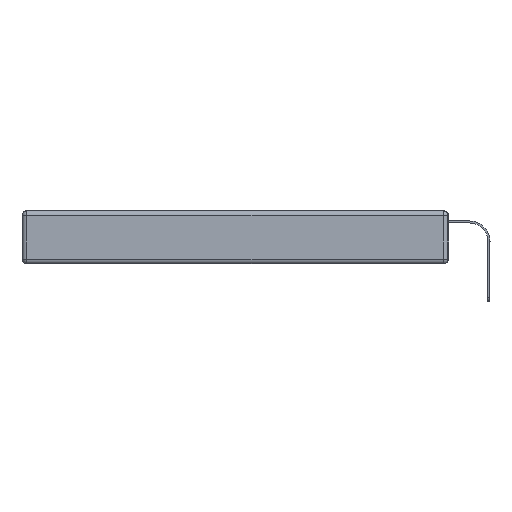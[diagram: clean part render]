
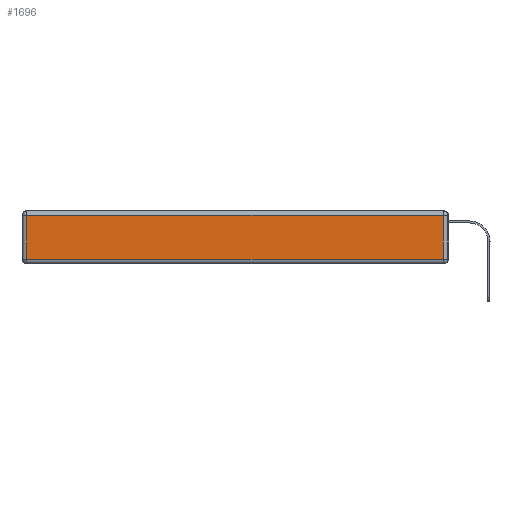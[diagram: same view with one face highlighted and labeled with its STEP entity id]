
A CAD part, left-side view. The second image highlights one B-rep face of the part: STEP entity #1696.
In plain terms, the highlighted planar face has unit normal (-1, 0, 0).
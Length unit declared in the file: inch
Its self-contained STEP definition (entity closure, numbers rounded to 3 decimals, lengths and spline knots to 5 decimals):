
#99 = VECTOR ( 'NONE', #16522, 39.37008 ) ;
#902 = VERTEX_POINT ( 'NONE', #2886 ) ;
#1073 = VECTOR ( 'NONE', #4844, 39.37008 ) ;
#1696 = ADVANCED_FACE ( 'NONE', ( #3199 ), #6491, .T. ) ;
#2133 = ORIENTED_EDGE ( 'NONE', *, *, #19074, .T. ) ;
#2134 = ORIENTED_EDGE ( 'NONE', *, *, #17268, .T. ) ;
#2862 = LINE ( 'NONE', #7171, #3297 ) ;
#2886 = CARTESIAN_POINT ( 'NONE',  ( 0., 2.72, -0.313 ) ) ;
#3199 = FACE_OUTER_BOUND ( 'NONE', #3744, .T. ) ;
#3297 = VECTOR ( 'NONE', #15186, 39.37008 ) ;
#3489 = CARTESIAN_POINT ( 'NONE',  ( 0., 0., -0.343 ) ) ;
#3527 = AXIS2_PLACEMENT_3D ( 'NONE', #3489, #15336, #9326 ) ;
#3744 = EDGE_LOOP ( 'NONE', ( #19801, #5757, #2133, #2134 ) ) ;
#4413 = CARTESIAN_POINT ( 'NONE',  ( 0., 0.03, -0.343 ) ) ;
#4572 = EDGE_CURVE ( 'NONE', #17485, #13929, #18167, .T. ) ;
#4844 = DIRECTION ( 'NONE',  ( 0., 1., 0. ) ) ;
#5757 = ORIENTED_EDGE ( 'NONE', *, *, #4572, .T. ) ;
#6167 = CARTESIAN_POINT ( 'NONE',  ( 0., 0.03, -0.313 ) ) ;
#6491 = PLANE ( 'NONE',  #3527 ) ;
#7171 = CARTESIAN_POINT ( 'NONE',  ( 0., 0., -0.313 ) ) ;
#7863 = LINE ( 'NONE', #15582, #1073 ) ;
#8714 = VECTOR ( 'NONE', #10742, 39.37008 ) ;
#9326 = DIRECTION ( 'NONE',  ( 0., 0., 1. ) ) ;
#10127 = CARTESIAN_POINT ( 'NONE',  ( 0., 2.72, -0.03 ) ) ;
#10742 = DIRECTION ( 'NONE',  ( 0., 0., 1. ) ) ;
#11923 = CARTESIAN_POINT ( 'NONE',  ( 0., 0.03, -0.03 ) ) ;
#12048 = CARTESIAN_POINT ( 'NONE',  ( 0., 2.72, -0.343 ) ) ;
#13929 = VERTEX_POINT ( 'NONE', #11923 ) ;
#15186 = DIRECTION ( 'NONE',  ( 0., -1., 0. ) ) ;
#15336 = DIRECTION ( 'NONE',  ( -1., 0., 0. ) ) ;
#15582 = CARTESIAN_POINT ( 'NONE',  ( 0., 2.75, -0.03 ) ) ;
#16522 = DIRECTION ( 'NONE',  ( 0., 0., -1. ) ) ;
#17268 = EDGE_CURVE ( 'NONE', #19556, #902, #18133, .T. ) ;
#17485 = VERTEX_POINT ( 'NONE', #6167 ) ;
#17638 = EDGE_CURVE ( 'NONE', #902, #17485, #2862, .T. ) ;
#18133 = LINE ( 'NONE', #12048, #99 ) ;
#18167 = LINE ( 'NONE', #4413, #8714 ) ;
#19074 = EDGE_CURVE ( 'NONE', #13929, #19556, #7863, .T. ) ;
#19556 = VERTEX_POINT ( 'NONE', #10127 ) ;
#19801 = ORIENTED_EDGE ( 'NONE', *, *, #17638, .T. ) ;
